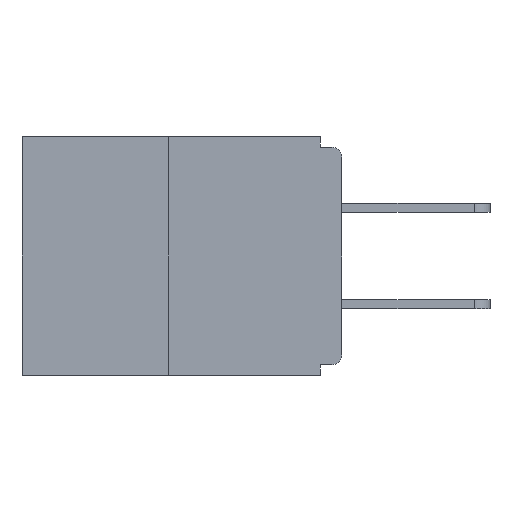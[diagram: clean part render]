
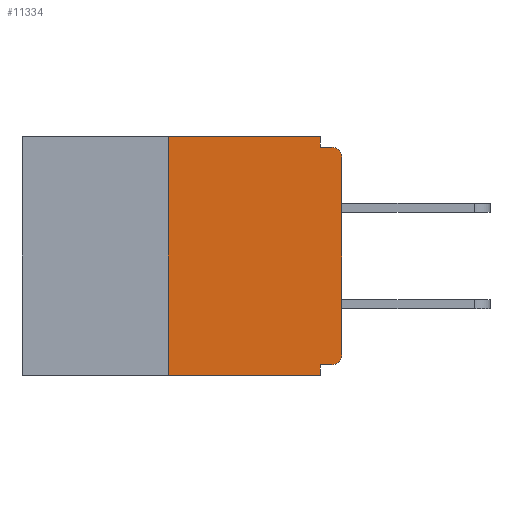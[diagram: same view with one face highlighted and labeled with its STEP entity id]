
A CAD part, left-side view. The second image highlights one B-rep face of the part: STEP entity #11334.
In plain terms, the highlighted planar face has unit normal (-1, 0, 0).
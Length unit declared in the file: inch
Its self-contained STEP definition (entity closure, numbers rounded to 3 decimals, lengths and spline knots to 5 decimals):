
#830 = LINE ( 'NONE', #29862, #25005 ) ;
#1176 = VECTOR ( 'NONE', #26489, 39.37008 ) ;
#1759 = DIRECTION ( 'NONE',  ( -1., 0., 0. ) ) ;
#2082 = VERTEX_POINT ( 'NONE', #8652 ) ;
#3196 = VECTOR ( 'NONE', #19303, 39.37008 ) ;
#3418 = DIRECTION ( 'NONE',  ( 0., 0., 1. ) ) ;
#3967 = VERTEX_POINT ( 'NONE', #26895 ) ;
#4135 = VECTOR ( 'NONE', #19182, 39.37008 ) ;
#4163 = ORIENTED_EDGE ( 'NONE', *, *, #25975, .F. ) ;
#4228 = LINE ( 'NONE', #20195, #29179 ) ;
#4489 = DIRECTION ( 'NONE',  ( 1., 0., 0. ) ) ;
#4639 = ORIENTED_EDGE ( 'NONE', *, *, #22907, .F. ) ;
#5144 = VERTEX_POINT ( 'NONE', #23704 ) ;
#6007 = VERTEX_POINT ( 'NONE', #17669 ) ;
#6267 = EDGE_CURVE ( 'NONE', #6007, #3967, #830, .T. ) ;
#6348 = CARTESIAN_POINT ( 'NONE',  ( 0., 0.031, 0. ) ) ;
#6372 = LINE ( 'NONE', #28945, #26187 ) ;
#6424 = ORIENTED_EDGE ( 'NONE', *, *, #22850, .T. ) ;
#6454 = VERTEX_POINT ( 'NONE', #17740 ) ;
#7956 = VERTEX_POINT ( 'NONE', #15136 ) ;
#8006 = CARTESIAN_POINT ( 'NONE',  ( 0., 0.031, -0.328 ) ) ;
#8165 = LINE ( 'NONE', #26194, #20613 ) ;
#8429 = CARTESIAN_POINT ( 'NONE',  ( 0., 0.015, -0.313 ) ) ;
#8652 = CARTESIAN_POINT ( 'NONE',  ( 0., 0.015, -0.328 ) ) ;
#9231 = AXIS2_PLACEMENT_3D ( 'NONE', #22529, #10590, #10888 ) ;
#9465 = DIRECTION ( 'NONE',  ( 0., -1., 0. ) ) ;
#9566 = ORIENTED_EDGE ( 'NONE', *, *, #11729, .T. ) ;
#9633 = AXIS2_PLACEMENT_3D ( 'NONE', #8429, #1759, #18164 ) ;
#10085 = ORIENTED_EDGE ( 'NONE', *, *, #17506, .F. ) ;
#10590 = DIRECTION ( 'NONE',  ( -1., 0., 0. ) ) ;
#10888 = DIRECTION ( 'NONE',  ( 0., 0., -1. ) ) ;
#11066 = CARTESIAN_POINT ( 'NONE',  ( 0., 0.25, 0. ) ) ;
#11334 = ADVANCED_FACE ( 'NONE', ( #14443 ), #25804, .F. ) ;
#11729 = EDGE_CURVE ( 'NONE', #2082, #24396, #16602, .T. ) ;
#11981 = DIRECTION ( 'NONE',  ( 0., 0., 1. ) ) ;
#12094 = EDGE_CURVE ( 'NONE', #26933, #5144, #27595, .T. ) ;
#12231 = CIRCLE ( 'NONE', #9231, 0.015 ) ;
#12366 = ORIENTED_EDGE ( 'NONE', *, *, #26423, .F. ) ;
#12593 = VERTEX_POINT ( 'NONE', #8006 ) ;
#14049 = DIRECTION ( 'NONE',  ( 0., 0., -1. ) ) ;
#14443 = FACE_OUTER_BOUND ( 'NONE', #17358, .T. ) ;
#15136 = CARTESIAN_POINT ( 'NONE',  ( 0., 0., -0.03 ) ) ;
#16236 = ORIENTED_EDGE ( 'NONE', *, *, #18488, .T. ) ;
#16602 = CIRCLE ( 'NONE', #9633, 0.015 ) ;
#17022 = VERTEX_POINT ( 'NONE', #11066 ) ;
#17048 = CARTESIAN_POINT ( 'NONE',  ( 0., 0., -0.328 ) ) ;
#17358 = EDGE_LOOP ( 'NONE', ( #10085, #20872, #22781, #4163, #12366, #9566, #16236, #6424, #26147, #4639 ) ) ;
#17506 = EDGE_CURVE ( 'NONE', #17022, #6454, #4228, .T. ) ;
#17669 = CARTESIAN_POINT ( 'NONE',  ( 0., 0.25, -0.343 ) ) ;
#17740 = CARTESIAN_POINT ( 'NONE',  ( 0., 0.031, 0. ) ) ;
#18164 = DIRECTION ( 'NONE',  ( 0., 0., -1. ) ) ;
#18488 = EDGE_CURVE ( 'NONE', #24396, #7956, #6372, .T. ) ;
#18535 = CARTESIAN_POINT ( 'NONE',  ( 0., 0.46, 0. ) ) ;
#19182 = DIRECTION ( 'NONE',  ( 0., 1., 0. ) ) ;
#19303 = DIRECTION ( 'NONE',  ( 0., 0., -1. ) ) ;
#19560 = LINE ( 'NONE', #17048, #4135 ) ;
#20195 = CARTESIAN_POINT ( 'NONE',  ( 0., 0.46, 0. ) ) ;
#20408 = LINE ( 'NONE', #21363, #3196 ) ;
#20613 = VECTOR ( 'NONE', #11981, 39.37008 ) ;
#20872 = ORIENTED_EDGE ( 'NONE', *, *, #23122, .F. ) ;
#21363 = CARTESIAN_POINT ( 'NONE',  ( 0., 0.031, -0.343 ) ) ;
#21762 = CARTESIAN_POINT ( 'NONE',  ( 0., 0., -0.015 ) ) ;
#22149 = AXIS2_PLACEMENT_3D ( 'NONE', #18535, #4489, #14049 ) ;
#22529 = CARTESIAN_POINT ( 'NONE',  ( 0., 0.015, -0.03 ) ) ;
#22781 = ORIENTED_EDGE ( 'NONE', *, *, #6267, .T. ) ;
#22850 = EDGE_CURVE ( 'NONE', #7956, #5144, #12231, .T. ) ;
#22907 = EDGE_CURVE ( 'NONE', #6454, #26933, #30180, .T. ) ;
#23122 = EDGE_CURVE ( 'NONE', #6007, #17022, #8165, .T. ) ;
#23348 = DIRECTION ( 'NONE',  ( 0., 0., -1. ) ) ;
#23606 = CARTESIAN_POINT ( 'NONE',  ( 0., 0., -0.313 ) ) ;
#23704 = CARTESIAN_POINT ( 'NONE',  ( 0., 0.015, -0.015 ) ) ;
#24396 = VERTEX_POINT ( 'NONE', #23606 ) ;
#25005 = VECTOR ( 'NONE', #9465, 39.37008 ) ;
#25804 = PLANE ( 'NONE',  #22149 ) ;
#25975 = EDGE_CURVE ( 'NONE', #12593, #3967, #20408, .T. ) ;
#26147 = ORIENTED_EDGE ( 'NONE', *, *, #12094, .F. ) ;
#26187 = VECTOR ( 'NONE', #3418, 39.37008 ) ;
#26194 = CARTESIAN_POINT ( 'NONE',  ( 0., 0.25, 0. ) ) ;
#26423 = EDGE_CURVE ( 'NONE', #2082, #12593, #19560, .T. ) ;
#26489 = DIRECTION ( 'NONE',  ( 0., -1., 0. ) ) ;
#26867 = VECTOR ( 'NONE', #23348, 39.37008 ) ;
#26895 = CARTESIAN_POINT ( 'NONE',  ( 0., 0.031, -0.343 ) ) ;
#26933 = VERTEX_POINT ( 'NONE', #30085 ) ;
#27595 = LINE ( 'NONE', #21762, #1176 ) ;
#28945 = CARTESIAN_POINT ( 'NONE',  ( 0., 0., 0. ) ) ;
#29179 = VECTOR ( 'NONE', #29733, 39.37008 ) ;
#29733 = DIRECTION ( 'NONE',  ( 0., -1., 0. ) ) ;
#29862 = CARTESIAN_POINT ( 'NONE',  ( 0., 0.46, -0.343 ) ) ;
#30085 = CARTESIAN_POINT ( 'NONE',  ( 0., 0.031, -0.015 ) ) ;
#30180 = LINE ( 'NONE', #6348, #26867 ) ;
